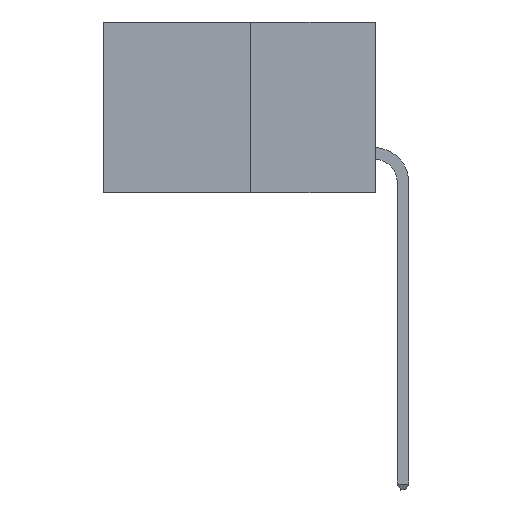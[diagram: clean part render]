
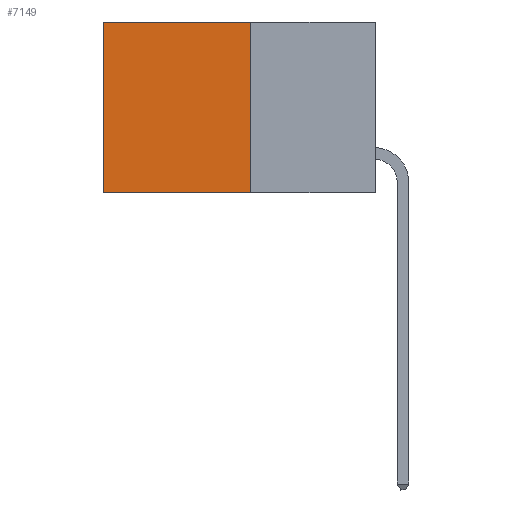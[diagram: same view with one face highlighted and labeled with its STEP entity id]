
A CAD part, left-side view. The second image highlights one B-rep face of the part: STEP entity #7149.
In plain terms, the highlighted planar face has unit normal (-1, 0, 0).
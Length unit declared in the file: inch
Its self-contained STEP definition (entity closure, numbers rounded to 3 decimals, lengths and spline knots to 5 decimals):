
#963 = EDGE_CURVE ( 'NONE', #23386, #15273, #8114, .T. ) ;
#1192 = VECTOR ( 'NONE', #19014, 39.37008 ) ;
#2373 = ORIENTED_EDGE ( 'NONE', *, *, #27419, .T. ) ;
#2387 = VERTEX_POINT ( 'NONE', #29574 ) ;
#3858 = LINE ( 'NONE', #20300, #25376 ) ;
#4701 = EDGE_CURVE ( 'NONE', #2387, #23386, #16381, .T. ) ;
#4757 = DIRECTION ( 'NONE',  ( 0., 0., -1. ) ) ;
#5602 = LINE ( 'NONE', #29384, #25492 ) ;
#6113 = DIRECTION ( 'NONE',  ( 0., 1., 0. ) ) ;
#6312 = DIRECTION ( 'NONE',  ( 0., 0., -1. ) ) ;
#6920 = FACE_OUTER_BOUND ( 'NONE', #13358, .T. ) ;
#7149 = ADVANCED_FACE ( 'NONE', ( #6920 ), #26534, .F. ) ;
#7799 = ORIENTED_EDGE ( 'NONE', *, *, #963, .F. ) ;
#8114 = LINE ( 'NONE', #26726, #1192 ) ;
#9459 = VECTOR ( 'NONE', #6312, 39.37008 ) ;
#12405 = VERTEX_POINT ( 'NONE', #25447 ) ;
#13358 = EDGE_LOOP ( 'NONE', ( #2373, #7799, #15708, #25596 ) ) ;
#13608 = DIRECTION ( 'NONE',  ( 0., 0., -1. ) ) ;
#14679 = CARTESIAN_POINT ( 'NONE',  ( 0.277, 0.27, -0.37 ) ) ;
#15273 = VERTEX_POINT ( 'NONE', #29759 ) ;
#15708 = ORIENTED_EDGE ( 'NONE', *, *, #4701, .F. ) ;
#15859 = EDGE_CURVE ( 'NONE', #2387, #12405, #5602, .T. ) ;
#16381 = LINE ( 'NONE', #24491, #9459 ) ;
#16757 = AXIS2_PLACEMENT_3D ( 'NONE', #21291, #29117, #13608 ) ;
#19014 = DIRECTION ( 'NONE',  ( 0., 1., 0. ) ) ;
#20300 = CARTESIAN_POINT ( 'NONE',  ( 0.277, 0.59, -0.37 ) ) ;
#21291 = CARTESIAN_POINT ( 'NONE',  ( 0.277, 0.27, -0.37 ) ) ;
#23386 = VERTEX_POINT ( 'NONE', #14679 ) ;
#24491 = CARTESIAN_POINT ( 'NONE',  ( 0.277, 0.27, -0.37 ) ) ;
#25376 = VECTOR ( 'NONE', #4757, 39.37008 ) ;
#25447 = CARTESIAN_POINT ( 'NONE',  ( 0.277, 0.59, 0. ) ) ;
#25492 = VECTOR ( 'NONE', #6113, 39.37008 ) ;
#25596 = ORIENTED_EDGE ( 'NONE', *, *, #15859, .T. ) ;
#26534 = PLANE ( 'NONE',  #16757 ) ;
#26726 = CARTESIAN_POINT ( 'NONE',  ( 0.277, 0.27, -0.37 ) ) ;
#27419 = EDGE_CURVE ( 'NONE', #12405, #15273, #3858, .T. ) ;
#29117 = DIRECTION ( 'NONE',  ( 1., 0., 0. ) ) ;
#29384 = CARTESIAN_POINT ( 'NONE',  ( 0.277, 0.27, 0. ) ) ;
#29574 = CARTESIAN_POINT ( 'NONE',  ( 0.277, 0.27, 0. ) ) ;
#29759 = CARTESIAN_POINT ( 'NONE',  ( 0.277, 0.59, -0.37 ) ) ;
